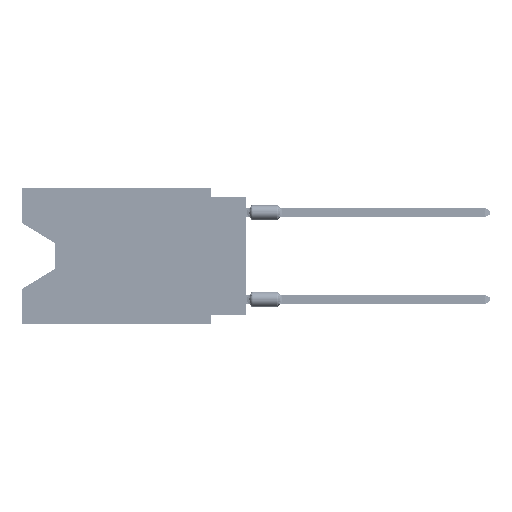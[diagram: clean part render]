
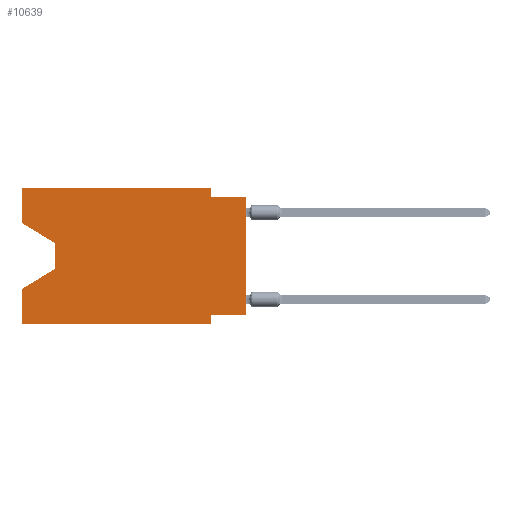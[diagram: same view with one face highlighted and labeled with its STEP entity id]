
A CAD part, left-side view. The second image highlights one B-rep face of the part: STEP entity #10639.
In plain terms, the highlighted planar face has unit normal (-1, 0, 0).
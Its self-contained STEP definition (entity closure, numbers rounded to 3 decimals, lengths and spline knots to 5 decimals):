
#876 = LINE ( 'NONE', #45654, #56073 ) ;
#4085 = VERTEX_POINT ( 'NONE', #40199 ) ;
#4486 = DIRECTION ( 'NONE',  ( 0., 0., -1. ) ) ;
#4886 = LINE ( 'NONE', #11814, #12941 ) ;
#5251 = VERTEX_POINT ( 'NONE', #43906 ) ;
#7820 = EDGE_CURVE ( 'NONE', #40509, #72503, #11049, .T. ) ;
#9225 = CARTESIAN_POINT ( 'NONE',  ( 0., 0., 0. ) ) ;
#9690 = ORIENTED_EDGE ( 'NONE', *, *, #71374, .F. ) ;
#10639 = ADVANCED_FACE ( 'NONE', ( #11562 ), #17226, .F. ) ;
#10986 = VECTOR ( 'NONE', #46255, 39.37008 ) ;
#11049 = LINE ( 'NONE', #64892, #27467 ) ;
#11494 = DIRECTION ( 'NONE',  ( 0., 0., -1. ) ) ;
#11510 = EDGE_LOOP ( 'NONE', ( #75091, #19747, #43075, #23142, #70067, #9690, #59767, #58926, #30583, #84943, #64096, #22299 ) ) ;
#11562 = FACE_OUTER_BOUND ( 'NONE', #11510, .T. ) ;
#11814 = CARTESIAN_POINT ( 'NONE',  ( 0., 0.1, 0. ) ) ;
#12686 = VERTEX_POINT ( 'NONE', #20743 ) ;
#12941 = VECTOR ( 'NONE', #17918, 39.37008 ) ;
#12978 = CARTESIAN_POINT ( 'NONE',  ( 0., 0.645, -0.28975 ) ) ;
#13704 = CARTESIAN_POINT ( 'NONE',  ( 0., 0.645, 0. ) ) ;
#16262 = EDGE_CURVE ( 'NONE', #76748, #71806, #4886, .T. ) ;
#16388 = CARTESIAN_POINT ( 'NONE',  ( 0., 0.645, -0.10025 ) ) ;
#17226 = PLANE ( 'NONE',  #26773 ) ;
#17918 = DIRECTION ( 'NONE',  ( 0., 0., -1. ) ) ;
#19747 = ORIENTED_EDGE ( 'NONE', *, *, #26435, .T. ) ;
#19784 = LINE ( 'NONE', #13704, #76805 ) ;
#19812 = DIRECTION ( 'NONE',  ( 0., -1., 0. ) ) ;
#20743 = CARTESIAN_POINT ( 'NONE',  ( 0., 0., -0.365 ) ) ;
#22299 = ORIENTED_EDGE ( 'NONE', *, *, #56863, .F. ) ;
#23142 = ORIENTED_EDGE ( 'NONE', *, *, #30335, .F. ) ;
#24304 = VECTOR ( 'NONE', #4486, 39.37008 ) ;
#24557 = CARTESIAN_POINT ( 'NONE',  ( 0., 0.55, -0.232 ) ) ;
#26435 = EDGE_CURVE ( 'NONE', #83932, #26900, #72639, .T. ) ;
#26773 = AXIS2_PLACEMENT_3D ( 'NONE', #30667, #49784, #57163 ) ;
#26900 = VERTEX_POINT ( 'NONE', #39509 ) ;
#27467 = VECTOR ( 'NONE', #64461, 39.37008 ) ;
#30335 = EDGE_CURVE ( 'NONE', #40509, #62966, #53178, .T. ) ;
#30583 = ORIENTED_EDGE ( 'NONE', *, *, #59017, .F. ) ;
#30667 = CARTESIAN_POINT ( 'NONE',  ( 0., 0.645, 0. ) ) ;
#31318 = VECTOR ( 'NONE', #36336, 39.37008 ) ;
#34449 = CARTESIAN_POINT ( 'NONE',  ( 0., 0., -0.365 ) ) ;
#36336 = DIRECTION ( 'NONE',  ( 0., -0.855, -0.519 ) ) ;
#38878 = CARTESIAN_POINT ( 'NONE',  ( 0., 0.645, 0. ) ) ;
#39509 = CARTESIAN_POINT ( 'NONE',  ( 0., 0.55, -0.232 ) ) ;
#40106 = DIRECTION ( 'NONE',  ( 0., 1., 0. ) ) ;
#40129 = CARTESIAN_POINT ( 'NONE',  ( 0., 0.55, -0.158 ) ) ;
#40199 = CARTESIAN_POINT ( 'NONE',  ( 0., 0.645, -0.10025 ) ) ;
#40509 = VERTEX_POINT ( 'NONE', #69101 ) ;
#41767 = DIRECTION ( 'NONE',  ( 0., 0., 1. ) ) ;
#41985 = CARTESIAN_POINT ( 'NONE',  ( 0., 0.1, -0.025 ) ) ;
#43075 = ORIENTED_EDGE ( 'NONE', *, *, #43972, .T. ) ;
#43906 = CARTESIAN_POINT ( 'NONE',  ( 0., 0., -0.025 ) ) ;
#43972 = EDGE_CURVE ( 'NONE', #26900, #62966, #84528, .T. ) ;
#44493 = LINE ( 'NONE', #71010, #84262 ) ;
#45654 = CARTESIAN_POINT ( 'NONE',  ( 0., 0.645, 0. ) ) ;
#46255 = DIRECTION ( 'NONE',  ( 0., 0., 1. ) ) ;
#46283 = DIRECTION ( 'NONE',  ( 0., -1., 0. ) ) ;
#47056 = LINE ( 'NONE', #34449, #70792 ) ;
#48093 = VECTOR ( 'NONE', #41767, 39.37008 ) ;
#48652 = CARTESIAN_POINT ( 'NONE',  ( 0., 0.1, -0.365 ) ) ;
#49784 = DIRECTION ( 'NONE',  ( 1., 0., 0. ) ) ;
#52297 = CARTESIAN_POINT ( 'NONE',  ( 0., 0.645, 0. ) ) ;
#53178 = LINE ( 'NONE', #38878, #10986 ) ;
#53515 = CARTESIAN_POINT ( 'NONE',  ( 0., 0.1, 0. ) ) ;
#56073 = VECTOR ( 'NONE', #73439, 39.37008 ) ;
#56106 = EDGE_CURVE ( 'NONE', #83996, #76748, #19784, .T. ) ;
#56863 = EDGE_CURVE ( 'NONE', #4085, #83996, #876, .T. ) ;
#57163 = DIRECTION ( 'NONE',  ( 0., 0., -1. ) ) ;
#57890 = CARTESIAN_POINT ( 'NONE',  ( 0., 0.55, -0.158 ) ) ;
#58013 = DIRECTION ( 'NONE',  ( 0., 0.855, -0.519 ) ) ;
#58926 = ORIENTED_EDGE ( 'NONE', *, *, #68642, .T. ) ;
#59017 = EDGE_CURVE ( 'NONE', #71806, #5251, #85862, .T. ) ;
#59442 = VERTEX_POINT ( 'NONE', #48652 ) ;
#59767 = ORIENTED_EDGE ( 'NONE', *, *, #67572, .F. ) ;
#60371 = EDGE_CURVE ( 'NONE', #4085, #83932, #75885, .T. ) ;
#62966 = VERTEX_POINT ( 'NONE', #12978 ) ;
#64096 = ORIENTED_EDGE ( 'NONE', *, *, #56106, .F. ) ;
#64457 = VECTOR ( 'NONE', #19812, 39.37008 ) ;
#64461 = DIRECTION ( 'NONE',  ( 0., -1., 0. ) ) ;
#64570 = CARTESIAN_POINT ( 'NONE',  ( 0., 0.1, -0.39 ) ) ;
#64892 = CARTESIAN_POINT ( 'NONE',  ( 0., 0.645, -0.39 ) ) ;
#67572 = EDGE_CURVE ( 'NONE', #12686, #59442, #47056, .T. ) ;
#68642 = EDGE_CURVE ( 'NONE', #12686, #5251, #73952, .T. ) ;
#69101 = CARTESIAN_POINT ( 'NONE',  ( 0., 0.645, -0.39 ) ) ;
#70067 = ORIENTED_EDGE ( 'NONE', *, *, #7820, .T. ) ;
#70792 = VECTOR ( 'NONE', #40106, 39.37008 ) ;
#71010 = CARTESIAN_POINT ( 'NONE',  ( 0., 0.1, -0.39 ) ) ;
#71374 = EDGE_CURVE ( 'NONE', #59442, #72503, #44493, .T. ) ;
#71806 = VERTEX_POINT ( 'NONE', #41985 ) ;
#72503 = VERTEX_POINT ( 'NONE', #64570 ) ;
#72639 = LINE ( 'NONE', #57890, #24304 ) ;
#73439 = DIRECTION ( 'NONE',  ( 0., 0., 1. ) ) ;
#73952 = LINE ( 'NONE', #9225, #48093 ) ;
#75091 = ORIENTED_EDGE ( 'NONE', *, *, #60371, .T. ) ;
#75885 = LINE ( 'NONE', #16388, #31318 ) ;
#76748 = VERTEX_POINT ( 'NONE', #53515 ) ;
#76805 = VECTOR ( 'NONE', #46283, 39.37008 ) ;
#77432 = VECTOR ( 'NONE', #58013, 39.37008 ) ;
#79328 = CARTESIAN_POINT ( 'NONE',  ( 0., 0., -0.025 ) ) ;
#83932 = VERTEX_POINT ( 'NONE', #40129 ) ;
#83996 = VERTEX_POINT ( 'NONE', #52297 ) ;
#84262 = VECTOR ( 'NONE', #11494, 39.37008 ) ;
#84528 = LINE ( 'NONE', #24557, #77432 ) ;
#84943 = ORIENTED_EDGE ( 'NONE', *, *, #16262, .F. ) ;
#85862 = LINE ( 'NONE', #79328, #64457 ) ;
